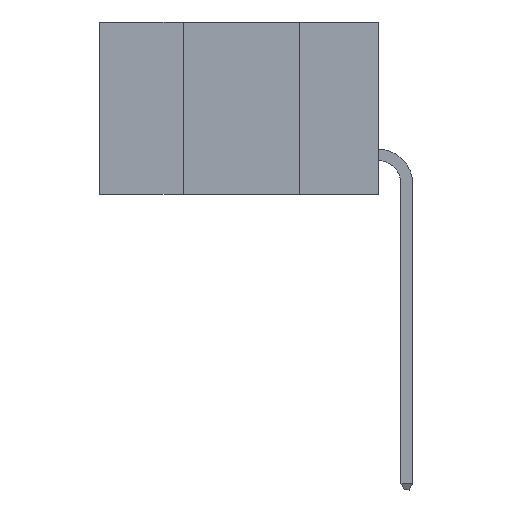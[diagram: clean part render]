
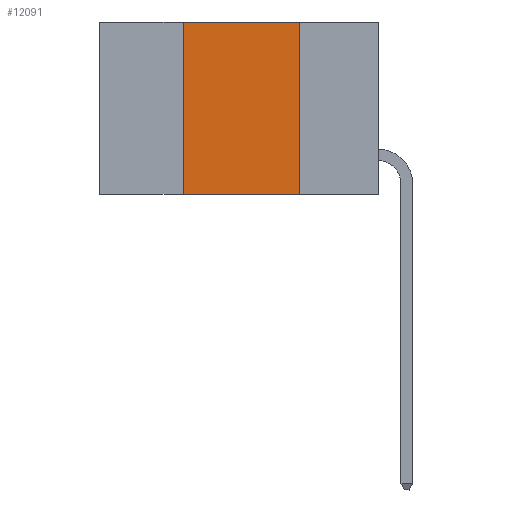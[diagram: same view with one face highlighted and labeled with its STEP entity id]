
A CAD part, left-side view. The second image highlights one B-rep face of the part: STEP entity #12091.
In plain terms, the highlighted planar face has unit normal (-1, 0, 0).
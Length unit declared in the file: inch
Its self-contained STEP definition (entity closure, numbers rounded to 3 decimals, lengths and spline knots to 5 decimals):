
#64 = ORIENTED_EDGE ( 'NONE', *, *, #10033, .T. ) ;
#731 = DIRECTION ( 'NONE',  ( 0., 0., 1. ) ) ;
#2534 = VERTEX_POINT ( 'NONE', #11968 ) ;
#2613 = EDGE_LOOP ( 'NONE', ( #12486, #4907, #10946, #64 ) ) ;
#2868 = AXIS2_PLACEMENT_3D ( 'NONE', #2948, #5319, #13174 ) ;
#2948 = CARTESIAN_POINT ( 'NONE',  ( 0., 0.6, 0. ) ) ;
#3036 = VECTOR ( 'NONE', #9730, 39.37008 ) ;
#3210 = VECTOR ( 'NONE', #7792, 39.37008 ) ;
#4136 = CARTESIAN_POINT ( 'NONE',  ( 0., 0.17, 0. ) ) ;
#4163 = VECTOR ( 'NONE', #731, 39.37008 ) ;
#4774 = VECTOR ( 'NONE', #8280, 39.37008 ) ;
#4907 = ORIENTED_EDGE ( 'NONE', *, *, #12176, .F. ) ;
#5319 = DIRECTION ( 'NONE',  ( 1., 0., 0. ) ) ;
#6001 = CARTESIAN_POINT ( 'NONE',  ( 0., 0.6, -0.37 ) ) ;
#6604 = VERTEX_POINT ( 'NONE', #4136 ) ;
#6654 = CARTESIAN_POINT ( 'NONE',  ( 0., 0.6, 0. ) ) ;
#7761 = CARTESIAN_POINT ( 'NONE',  ( 0., 0.42, 0. ) ) ;
#7792 = DIRECTION ( 'NONE',  ( 0., -1., 0. ) ) ;
#7833 = LINE ( 'NONE', #6001, #4774 ) ;
#8280 = DIRECTION ( 'NONE',  ( 0., -1., 0. ) ) ;
#8461 = FACE_OUTER_BOUND ( 'NONE', #2613, .T. ) ;
#8809 = VERTEX_POINT ( 'NONE', #12068 ) ;
#9518 = LINE ( 'NONE', #14108, #3036 ) ;
#9730 = DIRECTION ( 'NONE',  ( 0., 0., -1. ) ) ;
#10033 = EDGE_CURVE ( 'NONE', #8809, #2534, #7833, .T. ) ;
#10946 = ORIENTED_EDGE ( 'NONE', *, *, #11522, .F. ) ;
#11522 = EDGE_CURVE ( 'NONE', #8809, #12225, #12822, .T. ) ;
#11968 = CARTESIAN_POINT ( 'NONE',  ( 0., 0.17, -0.37 ) ) ;
#12068 = CARTESIAN_POINT ( 'NONE',  ( 0., 0.42, -0.37 ) ) ;
#12085 = PLANE ( 'NONE',  #2868 ) ;
#12091 = ADVANCED_FACE ( 'NONE', ( #8461 ), #12085, .F. ) ;
#12176 = EDGE_CURVE ( 'NONE', #12225, #6604, #12301, .T. ) ;
#12225 = VERTEX_POINT ( 'NONE', #12322 ) ;
#12301 = LINE ( 'NONE', #6654, #3210 ) ;
#12322 = CARTESIAN_POINT ( 'NONE',  ( 0., 0.42, 0. ) ) ;
#12486 = ORIENTED_EDGE ( 'NONE', *, *, #13710, .F. ) ;
#12822 = LINE ( 'NONE', #7761, #4163 ) ;
#13174 = DIRECTION ( 'NONE',  ( 0., 0., -1. ) ) ;
#13710 = EDGE_CURVE ( 'NONE', #6604, #2534, #9518, .T. ) ;
#14108 = CARTESIAN_POINT ( 'NONE',  ( 0., 0.17, 0. ) ) ;
